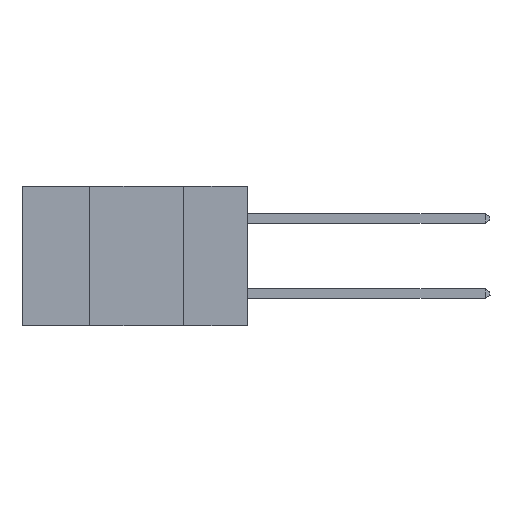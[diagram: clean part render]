
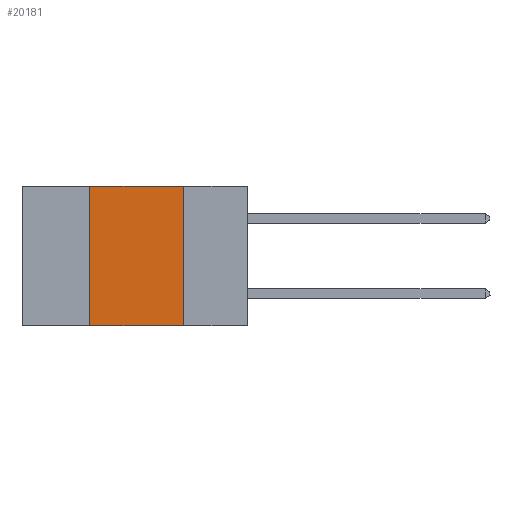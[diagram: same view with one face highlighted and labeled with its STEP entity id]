
A CAD part, left-side view. The second image highlights one B-rep face of the part: STEP entity #20181.
In plain terms, the highlighted planar face has unit normal (-1, 0, 0).
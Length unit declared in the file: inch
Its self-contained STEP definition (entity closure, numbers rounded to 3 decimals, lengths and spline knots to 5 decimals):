
#229 = ORIENTED_EDGE ( 'NONE', *, *, #18534, .F. ) ;
#330 = ORIENTED_EDGE ( 'NONE', *, *, #6571, .F. ) ;
#824 = LINE ( 'NONE', #3257, #18698 ) ;
#1202 = DIRECTION ( 'NONE',  ( 1., 0., 0. ) ) ;
#1493 = EDGE_CURVE ( 'NONE', #12163, #16149, #824, .T. ) ;
#1757 = FACE_OUTER_BOUND ( 'NONE', #8259, .T. ) ;
#2059 = CARTESIAN_POINT ( 'NONE',  ( 0., 0.17, -0.37 ) ) ;
#3257 = CARTESIAN_POINT ( 'NONE',  ( 0., 0.6, -0.37 ) ) ;
#3881 = LINE ( 'NONE', #15302, #13325 ) ;
#4952 = EDGE_CURVE ( 'NONE', #12163, #5293, #12564, .T. ) ;
#5117 = CARTESIAN_POINT ( 'NONE',  ( 0., 0.17, 0. ) ) ;
#5293 = VERTEX_POINT ( 'NONE', #20435 ) ;
#5651 = CARTESIAN_POINT ( 'NONE',  ( 0., 0.17, 0. ) ) ;
#5812 = CARTESIAN_POINT ( 'NONE',  ( 0., 0.42, 0. ) ) ;
#6571 = EDGE_CURVE ( 'NONE', #5293, #16806, #3881, .T. ) ;
#7747 = AXIS2_PLACEMENT_3D ( 'NONE', #18385, #1202, #8149 ) ;
#8149 = DIRECTION ( 'NONE',  ( 0., 0., -1. ) ) ;
#8259 = EDGE_LOOP ( 'NONE', ( #229, #330, #16351, #10155 ) ) ;
#8419 = DIRECTION ( 'NONE',  ( 0., -1., 0. ) ) ;
#9438 = DIRECTION ( 'NONE',  ( 0., 0., 1. ) ) ;
#10155 = ORIENTED_EDGE ( 'NONE', *, *, #1493, .T. ) ;
#12022 = VECTOR ( 'NONE', #9438, 39.37008 ) ;
#12163 = VERTEX_POINT ( 'NONE', #19368 ) ;
#12564 = LINE ( 'NONE', #5812, #12022 ) ;
#13325 = VECTOR ( 'NONE', #8419, 39.37008 ) ;
#15302 = CARTESIAN_POINT ( 'NONE',  ( 0., 0.6, 0. ) ) ;
#16149 = VERTEX_POINT ( 'NONE', #2059 ) ;
#16351 = ORIENTED_EDGE ( 'NONE', *, *, #4952, .F. ) ;
#16806 = VERTEX_POINT ( 'NONE', #5651 ) ;
#17266 = DIRECTION ( 'NONE',  ( 0., 0., -1. ) ) ;
#18385 = CARTESIAN_POINT ( 'NONE',  ( 0., 0.6, 0. ) ) ;
#18534 = EDGE_CURVE ( 'NONE', #16806, #16149, #20491, .T. ) ;
#18698 = VECTOR ( 'NONE', #20524, 39.37008 ) ;
#19368 = CARTESIAN_POINT ( 'NONE',  ( 0., 0.42, -0.37 ) ) ;
#20181 = ADVANCED_FACE ( 'NONE', ( #1757 ), #21998, .F. ) ;
#20435 = CARTESIAN_POINT ( 'NONE',  ( 0., 0.42, 0. ) ) ;
#20491 = LINE ( 'NONE', #5117, #21807 ) ;
#20524 = DIRECTION ( 'NONE',  ( 0., -1., 0. ) ) ;
#21807 = VECTOR ( 'NONE', #17266, 39.37008 ) ;
#21998 = PLANE ( 'NONE',  #7747 ) ;
